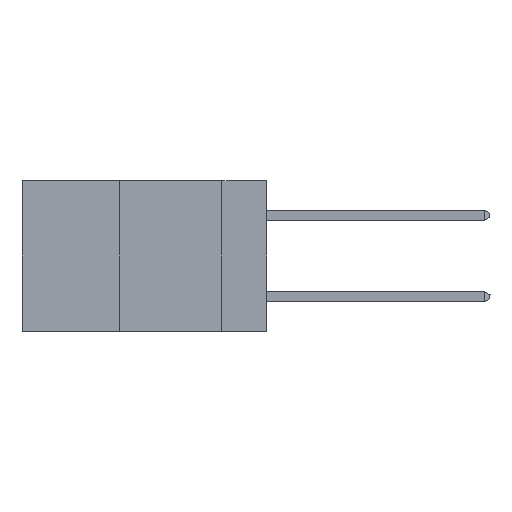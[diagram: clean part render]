
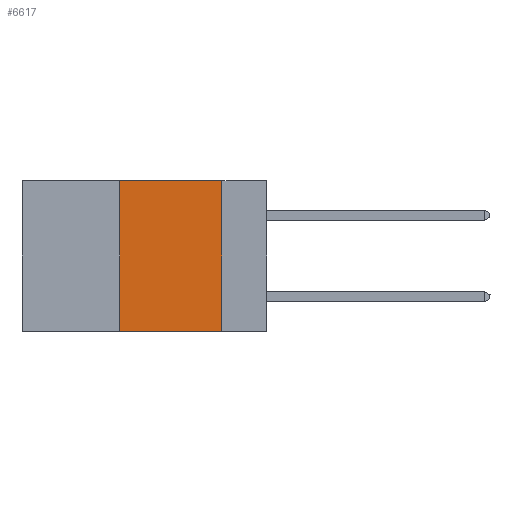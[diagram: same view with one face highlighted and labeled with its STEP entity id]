
A CAD part, left-side view. The second image highlights one B-rep face of the part: STEP entity #6617.
In plain terms, the highlighted planar face has unit normal (-1, 0, 0).
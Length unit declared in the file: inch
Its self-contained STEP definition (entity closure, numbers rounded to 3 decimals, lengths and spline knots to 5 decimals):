
#135 = CARTESIAN_POINT ( 'NONE',  ( 0., 0.6, 0. ) ) ;
#226 = VECTOR ( 'NONE', #11103, 39.37008 ) ;
#1786 = DIRECTION ( 'NONE',  ( 0., 0., -1. ) ) ;
#3019 = CARTESIAN_POINT ( 'NONE',  ( 0., 0.36, -0.37 ) ) ;
#3748 = ORIENTED_EDGE ( 'NONE', *, *, #14866, .F. ) ;
#4607 = LINE ( 'NONE', #16743, #7735 ) ;
#5007 = CARTESIAN_POINT ( 'NONE',  ( 0., 0.11, -0.37 ) ) ;
#5091 = ORIENTED_EDGE ( 'NONE', *, *, #7536, .T. ) ;
#5769 = VECTOR ( 'NONE', #12390, 39.37008 ) ;
#6608 = VECTOR ( 'NONE', #8335, 39.37008 ) ;
#6617 = ADVANCED_FACE ( 'NONE', ( #11379 ), #6693, .F. ) ;
#6693 = PLANE ( 'NONE',  #20157 ) ;
#7536 = EDGE_CURVE ( 'NONE', #9607, #17968, #4607, .T. ) ;
#7735 = VECTOR ( 'NONE', #11964, 39.37008 ) ;
#7842 = EDGE_LOOP ( 'NONE', ( #14680, #20596, #3748, #5091 ) ) ;
#8196 = LINE ( 'NONE', #11742, #6608 ) ;
#8294 = VERTEX_POINT ( 'NONE', #19346 ) ;
#8335 = DIRECTION ( 'NONE',  ( 0., 0., 1. ) ) ;
#9016 = LINE ( 'NONE', #9428, #226 ) ;
#9428 = CARTESIAN_POINT ( 'NONE',  ( 0., 0.11, 0. ) ) ;
#9607 = VERTEX_POINT ( 'NONE', #3019 ) ;
#9910 = CARTESIAN_POINT ( 'NONE',  ( 0., 0.11, 0. ) ) ;
#11103 = DIRECTION ( 'NONE',  ( 0., 0., -1. ) ) ;
#11379 = FACE_OUTER_BOUND ( 'NONE', #7842, .T. ) ;
#11742 = CARTESIAN_POINT ( 'NONE',  ( 0., 0.36, 0. ) ) ;
#11924 = EDGE_CURVE ( 'NONE', #8294, #17965, #20281, .T. ) ;
#11964 = DIRECTION ( 'NONE',  ( 0., -1., 0. ) ) ;
#12390 = DIRECTION ( 'NONE',  ( 0., -1., 0. ) ) ;
#12532 = CARTESIAN_POINT ( 'NONE',  ( 0., 0.6, 0. ) ) ;
#13466 = DIRECTION ( 'NONE',  ( 1., 0., 0. ) ) ;
#14619 = EDGE_CURVE ( 'NONE', #17965, #17968, #9016, .T. ) ;
#14680 = ORIENTED_EDGE ( 'NONE', *, *, #14619, .F. ) ;
#14866 = EDGE_CURVE ( 'NONE', #9607, #8294, #8196, .T. ) ;
#16743 = CARTESIAN_POINT ( 'NONE',  ( 0., 0.6, -0.37 ) ) ;
#17965 = VERTEX_POINT ( 'NONE', #9910 ) ;
#17968 = VERTEX_POINT ( 'NONE', #5007 ) ;
#19346 = CARTESIAN_POINT ( 'NONE',  ( 0., 0.36, 0. ) ) ;
#20157 = AXIS2_PLACEMENT_3D ( 'NONE', #135, #13466, #1786 ) ;
#20281 = LINE ( 'NONE', #12532, #5769 ) ;
#20596 = ORIENTED_EDGE ( 'NONE', *, *, #11924, .F. ) ;
